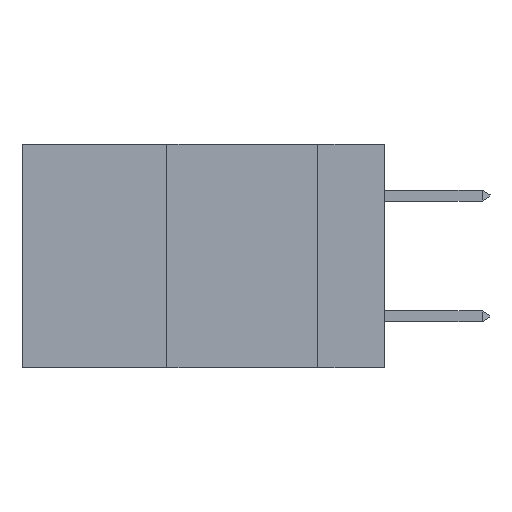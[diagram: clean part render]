
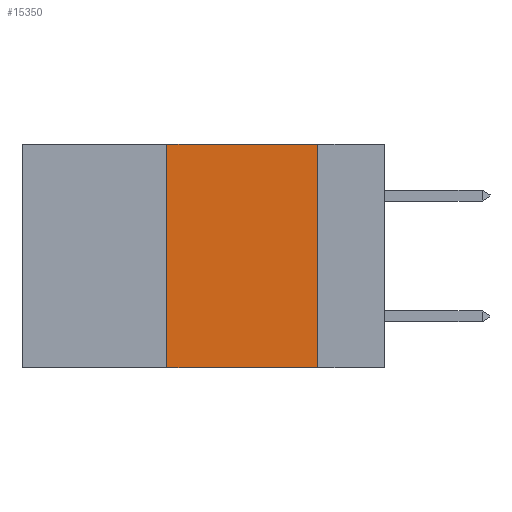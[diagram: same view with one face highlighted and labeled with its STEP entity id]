
A CAD part, left-side view. The second image highlights one B-rep face of the part: STEP entity #15350.
In plain terms, the highlighted planar face has unit normal (-1, 0, 0).
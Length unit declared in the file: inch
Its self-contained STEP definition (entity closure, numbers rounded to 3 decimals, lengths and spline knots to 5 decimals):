
#161 = EDGE_CURVE ( 'NONE', #27498, #10380, #22982, .T. ) ;
#977 = EDGE_CURVE ( 'NONE', #10380, #20997, #38540, .T. ) ;
#2052 = DIRECTION ( 'NONE',  ( 0., 0., -1. ) ) ;
#4446 = CARTESIAN_POINT ( 'NONE',  ( 0., 0.11, -0.37 ) ) ;
#4942 = DIRECTION ( 'NONE',  ( 0., -1., 0. ) ) ;
#5237 = EDGE_CURVE ( 'NONE', #20997, #36308, #38861, .T. ) ;
#6250 = PLANE ( 'NONE',  #7197 ) ;
#7197 = AXIS2_PLACEMENT_3D ( 'NONE', #15818, #28198, #18664 ) ;
#7533 = DIRECTION ( 'NONE',  ( 0., 0., 1. ) ) ;
#8041 = CARTESIAN_POINT ( 'NONE',  ( 0., 0.36, 0. ) ) ;
#8461 = ORIENTED_EDGE ( 'NONE', *, *, #977, .F. ) ;
#8814 = VECTOR ( 'NONE', #7533, 39.37008 ) ;
#9147 = CARTESIAN_POINT ( 'NONE',  ( 0., 0.36, -0.37 ) ) ;
#9485 = ORIENTED_EDGE ( 'NONE', *, *, #30819, .T. ) ;
#10380 = VERTEX_POINT ( 'NONE', #8041 ) ;
#10608 = VECTOR ( 'NONE', #4942, 39.37008 ) ;
#10801 = CARTESIAN_POINT ( 'NONE',  ( 0., 0.36, 0. ) ) ;
#14470 = VECTOR ( 'NONE', #20233, 39.37008 ) ;
#15350 = ADVANCED_FACE ( 'NONE', ( #31252 ), #6250, .F. ) ;
#15818 = CARTESIAN_POINT ( 'NONE',  ( 0., 0.6, 0. ) ) ;
#17475 = CARTESIAN_POINT ( 'NONE',  ( 0., 0.11, 0. ) ) ;
#18664 = DIRECTION ( 'NONE',  ( 0., 0., -1. ) ) ;
#18733 = VECTOR ( 'NONE', #2052, 39.37008 ) ;
#19069 = EDGE_LOOP ( 'NONE', ( #31504, #8461, #30355, #9485 ) ) ;
#20233 = DIRECTION ( 'NONE',  ( 0., -1., 0. ) ) ;
#20594 = LINE ( 'NONE', #23834, #10608 ) ;
#20997 = VERTEX_POINT ( 'NONE', #17475 ) ;
#22982 = LINE ( 'NONE', #10801, #8814 ) ;
#23834 = CARTESIAN_POINT ( 'NONE',  ( 0., 0.6, -0.37 ) ) ;
#27498 = VERTEX_POINT ( 'NONE', #9147 ) ;
#28198 = DIRECTION ( 'NONE',  ( 1., 0., 0. ) ) ;
#30355 = ORIENTED_EDGE ( 'NONE', *, *, #161, .F. ) ;
#30819 = EDGE_CURVE ( 'NONE', #27498, #36308, #20594, .T. ) ;
#31252 = FACE_OUTER_BOUND ( 'NONE', #19069, .T. ) ;
#31504 = ORIENTED_EDGE ( 'NONE', *, *, #5237, .F. ) ;
#35881 = CARTESIAN_POINT ( 'NONE',  ( 0., 0.6, 0. ) ) ;
#36308 = VERTEX_POINT ( 'NONE', #4446 ) ;
#38540 = LINE ( 'NONE', #35881, #14470 ) ;
#38660 = CARTESIAN_POINT ( 'NONE',  ( 0., 0.11, 0. ) ) ;
#38861 = LINE ( 'NONE', #38660, #18733 ) ;
